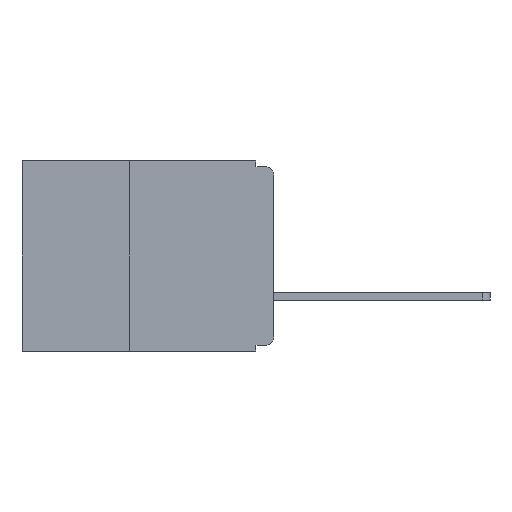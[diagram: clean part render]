
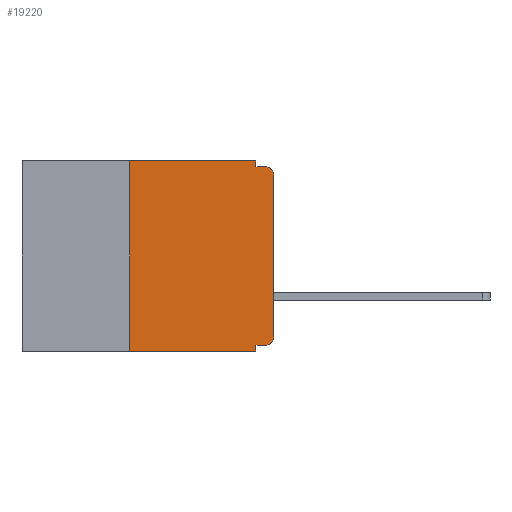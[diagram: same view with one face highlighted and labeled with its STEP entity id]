
A CAD part, left-side view. The second image highlights one B-rep face of the part: STEP entity #19220.
In plain terms, the highlighted planar face has unit normal (-1, 0, 0).
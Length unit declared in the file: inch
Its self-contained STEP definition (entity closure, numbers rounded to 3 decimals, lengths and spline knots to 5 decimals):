
#133 = DIRECTION ( 'NONE',  ( 0., 0., 1. ) ) ;
#190 = CARTESIAN_POINT ( 'NONE',  ( 0., 0.25, -0.33 ) ) ;
#807 = ORIENTED_EDGE ( 'NONE', *, *, #6075, .F. ) ;
#986 = DIRECTION ( 'NONE',  ( 0., 0., -1. ) ) ;
#1190 = LINE ( 'NONE', #13543, #14554 ) ;
#1326 = ORIENTED_EDGE ( 'NONE', *, *, #11580, .T. ) ;
#1473 = ORIENTED_EDGE ( 'NONE', *, *, #2710, .T. ) ;
#2009 = VERTEX_POINT ( 'NONE', #16166 ) ;
#2394 = LINE ( 'NONE', #4706, #19776 ) ;
#2526 = LINE ( 'NONE', #2897, #20449 ) ;
#2710 = EDGE_CURVE ( 'NONE', #15747, #15026, #4757, .T. ) ;
#2764 = VERTEX_POINT ( 'NONE', #19196 ) ;
#2897 = CARTESIAN_POINT ( 'NONE',  ( 0., 0.031, 0. ) ) ;
#3169 = LINE ( 'NONE', #21961, #11372 ) ;
#3204 = VECTOR ( 'NONE', #20834, 39.37008 ) ;
#3232 = AXIS2_PLACEMENT_3D ( 'NONE', #19783, #19742, #19711 ) ;
#3545 = ORIENTED_EDGE ( 'NONE', *, *, #14977, .T. ) ;
#4011 = CARTESIAN_POINT ( 'NONE',  ( 0., 0.015, -0.305 ) ) ;
#4222 = CARTESIAN_POINT ( 'NONE',  ( 0., 0.015, -0.32 ) ) ;
#4419 = CARTESIAN_POINT ( 'NONE',  ( 0., 0.437, 0. ) ) ;
#4506 = VERTEX_POINT ( 'NONE', #5720 ) ;
#4706 = CARTESIAN_POINT ( 'NONE',  ( 0., 0., -0.01 ) ) ;
#4757 = CIRCLE ( 'NONE', #3232, 0.015 ) ;
#4962 = FACE_OUTER_BOUND ( 'NONE', #5884, .T. ) ;
#5359 = ORIENTED_EDGE ( 'NONE', *, *, #11847, .F. ) ;
#5720 = CARTESIAN_POINT ( 'NONE',  ( 0., 0., -0.305 ) ) ;
#5804 = DIRECTION ( 'NONE',  ( 0., 0., -1. ) ) ;
#5884 = EDGE_LOOP ( 'NONE', ( #3545, #1473, #807, #9975, #22465, #5359, #1326, #7410, #14724, #17721 ) ) ;
#6027 = CARTESIAN_POINT ( 'NONE',  ( 0., 0.031, -0.32 ) ) ;
#6075 = EDGE_CURVE ( 'NONE', #19274, #15026, #2394, .T. ) ;
#6099 = DIRECTION ( 'NONE',  ( 0., 0., 1. ) ) ;
#6258 = LINE ( 'NONE', #19185, #20042 ) ;
#6410 = DIRECTION ( 'NONE',  ( 0., -1., 0. ) ) ;
#6570 = DIRECTION ( 'NONE',  ( 0., 1., 0. ) ) ;
#6660 = EDGE_CURVE ( 'NONE', #17321, #2764, #3169, .T. ) ;
#6956 = VERTEX_POINT ( 'NONE', #190 ) ;
#6998 = CARTESIAN_POINT ( 'NONE',  ( 0., 0.437, 0. ) ) ;
#7410 = ORIENTED_EDGE ( 'NONE', *, *, #6660, .F. ) ;
#7423 = VERTEX_POINT ( 'NONE', #4222 ) ;
#8210 = CARTESIAN_POINT ( 'NONE',  ( 0., 0.031, -0.01 ) ) ;
#8288 = EDGE_CURVE ( 'NONE', #7423, #17321, #1190, .T. ) ;
#8641 = AXIS2_PLACEMENT_3D ( 'NONE', #4419, #11427, #986 ) ;
#9504 = EDGE_CURVE ( 'NONE', #14553, #19274, #2526, .T. ) ;
#9935 = VECTOR ( 'NONE', #6099, 39.37008 ) ;
#9975 = ORIENTED_EDGE ( 'NONE', *, *, #9504, .F. ) ;
#10489 = LINE ( 'NONE', #19923, #9935 ) ;
#11145 = VECTOR ( 'NONE', #6410, 39.37008 ) ;
#11372 = VECTOR ( 'NONE', #16850, 39.37008 ) ;
#11404 = LINE ( 'NONE', #6998, #3204 ) ;
#11427 = DIRECTION ( 'NONE',  ( 1., 0., 0. ) ) ;
#11580 = EDGE_CURVE ( 'NONE', #6956, #2764, #15749, .T. ) ;
#11711 = DIRECTION ( 'NONE',  ( 0., -1., 0. ) ) ;
#11811 = EDGE_CURVE ( 'NONE', #2009, #14553, #11404, .T. ) ;
#11847 = EDGE_CURVE ( 'NONE', #6956, #2009, #6258, .T. ) ;
#13543 = CARTESIAN_POINT ( 'NONE',  ( 0., 0., -0.32 ) ) ;
#13649 = CIRCLE ( 'NONE', #18625, 0.015 ) ;
#14553 = VERTEX_POINT ( 'NONE', #17027 ) ;
#14554 = VECTOR ( 'NONE', #6570, 39.37008 ) ;
#14724 = ORIENTED_EDGE ( 'NONE', *, *, #8288, .F. ) ;
#14845 = PLANE ( 'NONE',  #8641 ) ;
#14977 = EDGE_CURVE ( 'NONE', #4506, #15747, #10489, .T. ) ;
#15026 = VERTEX_POINT ( 'NONE', #20001 ) ;
#15747 = VERTEX_POINT ( 'NONE', #20528 ) ;
#15749 = LINE ( 'NONE', #18530, #11145 ) ;
#16166 = CARTESIAN_POINT ( 'NONE',  ( 0., 0.25, 0. ) ) ;
#16189 = DIRECTION ( 'NONE',  ( -1., 0., 0. ) ) ;
#16850 = DIRECTION ( 'NONE',  ( 0., 0., -1. ) ) ;
#17027 = CARTESIAN_POINT ( 'NONE',  ( 0., 0.031, 0. ) ) ;
#17321 = VERTEX_POINT ( 'NONE', #6027 ) ;
#17721 = ORIENTED_EDGE ( 'NONE', *, *, #19652, .T. ) ;
#18530 = CARTESIAN_POINT ( 'NONE',  ( 0., 0.437, -0.33 ) ) ;
#18625 = AXIS2_PLACEMENT_3D ( 'NONE', #4011, #16189, #5804 ) ;
#18631 = DIRECTION ( 'NONE',  ( 0., 0., -1. ) ) ;
#19185 = CARTESIAN_POINT ( 'NONE',  ( 0., 0.25, -0.33 ) ) ;
#19196 = CARTESIAN_POINT ( 'NONE',  ( 0., 0.031, -0.33 ) ) ;
#19220 = ADVANCED_FACE ( 'NONE', ( #4962 ), #14845, .F. ) ;
#19274 = VERTEX_POINT ( 'NONE', #8210 ) ;
#19652 = EDGE_CURVE ( 'NONE', #7423, #4506, #13649, .T. ) ;
#19711 = DIRECTION ( 'NONE',  ( 0., 0., -1. ) ) ;
#19742 = DIRECTION ( 'NONE',  ( -1., 0., 0. ) ) ;
#19776 = VECTOR ( 'NONE', #11711, 39.37008 ) ;
#19783 = CARTESIAN_POINT ( 'NONE',  ( 0., 0.015, -0.025 ) ) ;
#19923 = CARTESIAN_POINT ( 'NONE',  ( 0., 0., 0. ) ) ;
#20001 = CARTESIAN_POINT ( 'NONE',  ( 0., 0.015, -0.01 ) ) ;
#20042 = VECTOR ( 'NONE', #133, 39.37008 ) ;
#20449 = VECTOR ( 'NONE', #18631, 39.37008 ) ;
#20528 = CARTESIAN_POINT ( 'NONE',  ( 0., 0., -0.025 ) ) ;
#20834 = DIRECTION ( 'NONE',  ( 0., -1., 0. ) ) ;
#21961 = CARTESIAN_POINT ( 'NONE',  ( 0., 0.031, -0.33 ) ) ;
#22465 = ORIENTED_EDGE ( 'NONE', *, *, #11811, .F. ) ;
